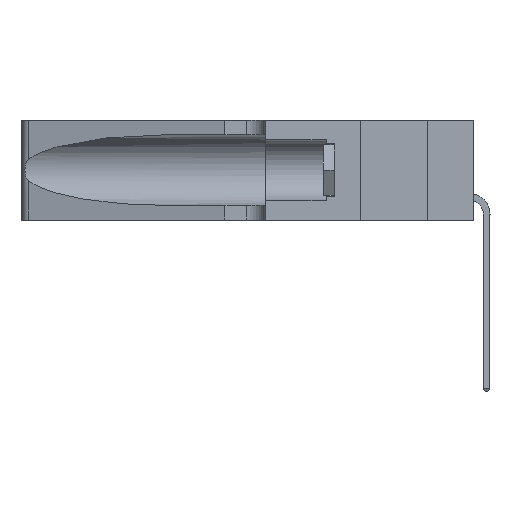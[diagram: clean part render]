
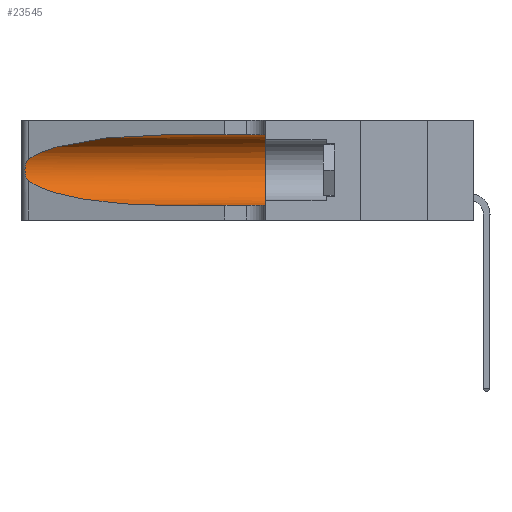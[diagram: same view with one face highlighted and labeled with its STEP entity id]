
A CAD part, left-side view. The second image highlights one B-rep face of the part: STEP entity #23545.
In plain terms, the highlighted cylindrical face has radius 3.308 mm (diameter 6.617 mm), a partial arc.
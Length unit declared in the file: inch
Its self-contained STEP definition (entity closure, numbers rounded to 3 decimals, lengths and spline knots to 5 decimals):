
#129 = CARTESIAN_POINT ( 'NONE',  ( 0.25787, 1.23484, 0.2124 ) ) ;
#395 = ORIENTED_EDGE ( 'NONE', *, *, #24518, .T. ) ;
#633 = CARTESIAN_POINT ( 'NONE',  ( 0.2373, 1.15595, 0.08982 ) ) ;
#986 = VERTEX_POINT ( 'NONE', #23356 ) ;
#1483 = CARTESIAN_POINT ( 'NONE',  ( 0.1305, 0.72297, 0.31525 ) ) ;
#1616 = EDGE_LOOP ( 'NONE', ( #13996, #8150, #395, #14089, #16431, #17990 ) ) ;
#2264 = CARTESIAN_POINT ( 'NONE',  ( 0.26075, 1.23896, 0.178 ) ) ;
#3314 = CARTESIAN_POINT ( 'NONE',  ( 0.25487, 1.22718, 0.22369 ) ) ;
#3922 = DIRECTION ( 'NONE',  ( 0., 1., 0. ) ) ;
#4339 = CARTESIAN_POINT ( 'NONE',  ( 0.25555, 1.22994, 0.2215 ) ) ;
#4403 = EDGE_CURVE ( 'NONE', #21440, #24362, #21846, .T. ) ;
#4473 = CARTESIAN_POINT ( 'NONE',  ( 0.1305, 0.72297, 0.05475 ) ) ;
#4531 = CARTESIAN_POINT ( 'NONE',  ( 0.25487, 1.22718, 0.14631 ) ) ;
#4656 = FACE_OUTER_BOUND ( 'NONE', #1616, .T. ) ;
#4843 = LINE ( 'NONE', #24115, #12732 ) ;
#5373 = EDGE_CURVE ( 'NONE', #986, #6960, #9464, .T. ) ;
#5635 = DIRECTION ( 'NONE',  ( 0., 0., -1. ) ) ;
#6433 = CARTESIAN_POINT ( 'NONE',  ( 0.25789, 1.23486, 0.15765 ) ) ;
#6450 = AXIS2_PLACEMENT_3D ( 'NONE', #20536, #3922, #16415 ) ;
#6608 = CARTESIAN_POINT ( 'NONE',  ( 0.25639, 1.23184, 0.21858 ) ) ;
#6734 = EDGE_CURVE ( 'NONE', #6960, #12859, #25270, .T. ) ;
#6960 = VERTEX_POINT ( 'NONE', #21294 ) ;
#7686 = CARTESIAN_POINT ( 'NONE',  ( 0.1305, 1.61858, 0.05475 ) ) ;
#8150 = ORIENTED_EDGE ( 'NONE', *, *, #6734, .T. ) ;
#9464 =( BOUNDED_CURVE ( )  B_SPLINE_CURVE ( 3, ( #1483, #11664, #26361, #3314 ),
 .UNSPECIFIED., .F., .F. ) 
 B_SPLINE_CURVE_WITH_KNOTS ( ( 4, 4 ),
 ( 1.5708, 2.84003 ),
 .UNSPECIFIED. ) 
 CURVE ( )  GEOMETRIC_REPRESENTATION_ITEM ( )  RATIONAL_B_SPLINE_CURVE ( ( 1., 0.87, 0.87, 1. ) ) 
 REPRESENTATION_ITEM ( '' )  );
#9797 = DIRECTION ( 'NONE',  ( 0., -1., 0. ) ) ;
#10252 = CARTESIAN_POINT ( 'NONE',  ( 0.1305, 0.72297, 0.05475 ) ) ;
#10571 = CARTESIAN_POINT ( 'NONE',  ( 0.26075, 1.23896, 0.19203 ) ) ;
#10660 = VECTOR ( 'NONE', #9797, 39.37008 ) ;
#11664 = CARTESIAN_POINT ( 'NONE',  ( 0.18966, 0.96281, 0.31525 ) ) ;
#12728 = CARTESIAN_POINT ( 'NONE',  ( 0.25487, 1.22718, 0.22369 ) ) ;
#12732 = VECTOR ( 'NONE', #23934, 39.37008 ) ;
#12859 = VERTEX_POINT ( 'NONE', #14106 ) ;
#13139 = CARTESIAN_POINT ( 'NONE',  ( 0.25487, 1.22718, 0.14631 ) ) ;
#13996 = ORIENTED_EDGE ( 'NONE', *, *, #5373, .T. ) ;
#14089 = ORIENTED_EDGE ( 'NONE', *, *, #4403, .T. ) ;
#14106 = CARTESIAN_POINT ( 'NONE',  ( 0.25487, 1.22718, 0.14631 ) ) ;
#14274 = DIRECTION ( 'NONE',  ( 0., -1., 0. ) ) ;
#14432 = CARTESIAN_POINT ( 'NONE',  ( 0.1305, 0.35, 0.05475 ) ) ;
#14825 = CARTESIAN_POINT ( 'NONE',  ( 0.26018, 1.23835, 0.19895 ) ) ;
#15198 = CIRCLE ( 'NONE', #6450, 0.13025 ) ;
#16415 = DIRECTION ( 'NONE',  ( 0., 0., 1. ) ) ;
#16431 = ORIENTED_EDGE ( 'NONE', *, *, #17506, .F. ) ;
#16976 = CARTESIAN_POINT ( 'NONE',  ( 0.26017, 1.23833, 0.17102 ) ) ;
#17506 = EDGE_CURVE ( 'NONE', #17660, #24362, #15198, .T. ) ;
#17660 = VERTEX_POINT ( 'NONE', #21508 ) ;
#17990 = ORIENTED_EDGE ( 'NONE', *, *, #20593, .F. ) ;
#18255 = CARTESIAN_POINT ( 'NONE',  ( 0.1305, 1.61858, 0.185 ) ) ;
#19056 = CARTESIAN_POINT ( 'NONE',  ( 0.25856, 1.23593, 0.16098 ) ) ;
#19447 = CARTESIAN_POINT ( 'NONE',  ( 0.18966, 0.96281, 0.05475 ) ) ;
#19453 = AXIS2_PLACEMENT_3D ( 'NONE', #18255, #14274, #5635 ) ;
#20536 = CARTESIAN_POINT ( 'NONE',  ( 0.1305, 0.35, 0.185 ) ) ;
#20593 = EDGE_CURVE ( 'NONE', #986, #17660, #4843, .T. ) ;
#21294 = CARTESIAN_POINT ( 'NONE',  ( 0.25487, 1.22718, 0.22369 ) ) ;
#21440 = VERTEX_POINT ( 'NONE', #10252 ) ;
#21508 = CARTESIAN_POINT ( 'NONE',  ( 0.1305, 0.35, 0.31525 ) ) ;
#21846 = LINE ( 'NONE', #7686, #10660 ) ;
#23036 = CYLINDRICAL_SURFACE ( 'NONE', #19453, 0.13025 ) ;
#23077 = CARTESIAN_POINT ( 'NONE',  ( 0.25555, 1.22993, 0.14849 ) ) ;
#23348 = CARTESIAN_POINT ( 'NONE',  ( 0.25854, 1.2359, 0.20912 ) ) ;
#23356 = CARTESIAN_POINT ( 'NONE',  ( 0.1305, 0.72297, 0.31525 ) ) ;
#23545 = ADVANCED_FACE ( 'NONE', ( #4656 ), #23036, .F. ) ;
#23934 = DIRECTION ( 'NONE',  ( 0., -1., 0. ) ) ;
#24115 = CARTESIAN_POINT ( 'NONE',  ( 0.1305, 1.61858, 0.31525 ) ) ;
#24362 = VERTEX_POINT ( 'NONE', #14432 ) ;
#24451 =( BOUNDED_CURVE ( )  B_SPLINE_CURVE ( 3, ( #13139, #633, #19447, #4473 ),
 .UNSPECIFIED., .F., .T. ) 
 B_SPLINE_CURVE_WITH_KNOTS ( ( 4, 4 ),
 ( 3.44316, 4.71239 ),
 .UNSPECIFIED. ) 
 CURVE ( )  GEOMETRIC_REPRESENTATION_ITEM ( )  RATIONAL_B_SPLINE_CURVE ( ( 1., 0.87, 0.87, 1. ) ) 
 REPRESENTATION_ITEM ( '' )  );
#24518 = EDGE_CURVE ( 'NONE', #12859, #21440, #24451, .T. ) ;
#25270 = B_SPLINE_CURVE_WITH_KNOTS ( 'NONE', 3,
 ( #12728, #4339, #6608, #129, #23348, #14825, #10571, #2264, #16976, #19056, #6433, #25445, #23077, #4531 ),
 .UNSPECIFIED., .F., .F.,
 ( 4, 2, 2, 2, 2, 2, 4 ),
 ( 0., 0.00027, 0.00053, 0.00107, 0.0016, 0.00187, 0.00214 ),
 .UNSPECIFIED. ) ;
#25445 = CARTESIAN_POINT ( 'NONE',  ( 0.25639, 1.23186, 0.15144 ) ) ;
#26361 = CARTESIAN_POINT ( 'NONE',  ( 0.2373, 1.15595, 0.28018 ) ) ;
